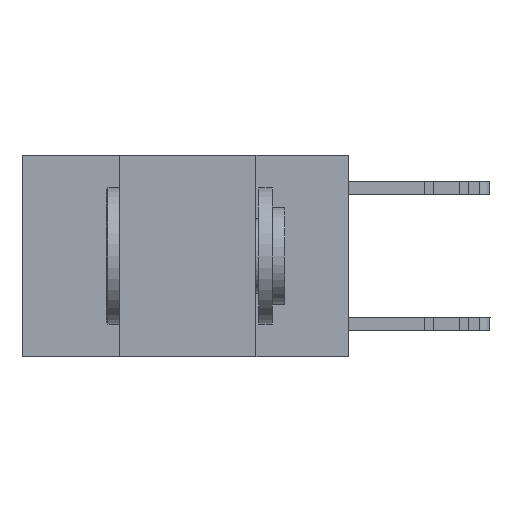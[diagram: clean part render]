
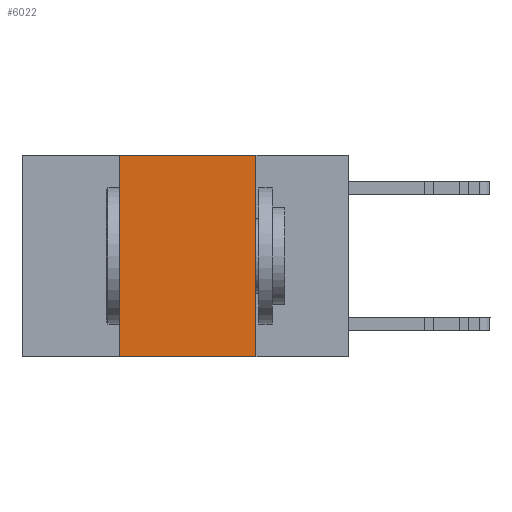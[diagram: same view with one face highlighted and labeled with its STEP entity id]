
A CAD part, left-side view. The second image highlights one B-rep face of the part: STEP entity #6022.
In plain terms, the highlighted planar face has unit normal (-1, 0, 0).
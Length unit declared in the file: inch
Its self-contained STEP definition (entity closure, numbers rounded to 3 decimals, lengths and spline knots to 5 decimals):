
#36 = VERTEX_POINT ( 'NONE', #921 ) ;
#921 = CARTESIAN_POINT ( 'NONE',  ( 0., 0.17, 0. ) ) ;
#2016 = DIRECTION ( 'NONE',  ( 0., 0., -1. ) ) ;
#2058 = CARTESIAN_POINT ( 'NONE',  ( 0., 0.17, 0. ) ) ;
#2634 = VERTEX_POINT ( 'NONE', #12006 ) ;
#2759 = VERTEX_POINT ( 'NONE', #30966 ) ;
#4236 = FACE_OUTER_BOUND ( 'NONE', #15179, .T. ) ;
#6022 = ADVANCED_FACE ( 'NONE', ( #4236 ), #15856, .F. ) ;
#6220 = LINE ( 'NONE', #8512, #25813 ) ;
#6436 = LINE ( 'NONE', #31364, #18835 ) ;
#8105 = CARTESIAN_POINT ( 'NONE',  ( 0., 0.42, 0. ) ) ;
#8512 = CARTESIAN_POINT ( 'NONE',  ( 0., 0.6, 0. ) ) ;
#10465 = EDGE_CURVE ( 'NONE', #36, #2634, #16620, .T. ) ;
#11694 = EDGE_CURVE ( 'NONE', #2759, #23721, #25556, .T. ) ;
#12006 = CARTESIAN_POINT ( 'NONE',  ( 0., 0.17, -0.37 ) ) ;
#13206 = ORIENTED_EDGE ( 'NONE', *, *, #20528, .T. ) ;
#14497 = DIRECTION ( 'NONE',  ( 0., -1., 0. ) ) ;
#15179 = EDGE_LOOP ( 'NONE', ( #21268, #18571, #20539, #13206 ) ) ;
#15543 = DIRECTION ( 'NONE',  ( 0., 0., -1. ) ) ;
#15612 = DIRECTION ( 'NONE',  ( 1., 0., 0. ) ) ;
#15856 = PLANE ( 'NONE',  #17256 ) ;
#15889 = CARTESIAN_POINT ( 'NONE',  ( 0., 0.6, 0. ) ) ;
#16482 = VECTOR ( 'NONE', #2016, 39.37008 ) ;
#16620 = LINE ( 'NONE', #2058, #16482 ) ;
#17256 = AXIS2_PLACEMENT_3D ( 'NONE', #15889, #15612, #15543 ) ;
#18571 = ORIENTED_EDGE ( 'NONE', *, *, #24380, .F. ) ;
#18835 = VECTOR ( 'NONE', #14497, 39.37008 ) ;
#20528 = EDGE_CURVE ( 'NONE', #2759, #2634, #6436, .T. ) ;
#20539 = ORIENTED_EDGE ( 'NONE', *, *, #11694, .F. ) ;
#21268 = ORIENTED_EDGE ( 'NONE', *, *, #10465, .F. ) ;
#23696 = DIRECTION ( 'NONE',  ( 0., 0., 1. ) ) ;
#23721 = VERTEX_POINT ( 'NONE', #8105 ) ;
#23872 = CARTESIAN_POINT ( 'NONE',  ( 0., 0.42, 0. ) ) ;
#24380 = EDGE_CURVE ( 'NONE', #23721, #36, #6220, .T. ) ;
#25500 = VECTOR ( 'NONE', #23696, 39.37008 ) ;
#25556 = LINE ( 'NONE', #23872, #25500 ) ;
#25627 = DIRECTION ( 'NONE',  ( 0., -1., 0. ) ) ;
#25813 = VECTOR ( 'NONE', #25627, 39.37008 ) ;
#30966 = CARTESIAN_POINT ( 'NONE',  ( 0., 0.42, -0.37 ) ) ;
#31364 = CARTESIAN_POINT ( 'NONE',  ( 0., 0.6, -0.37 ) ) ;
